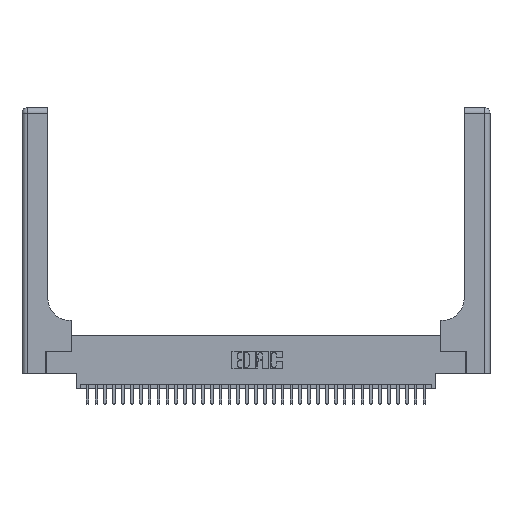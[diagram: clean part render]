
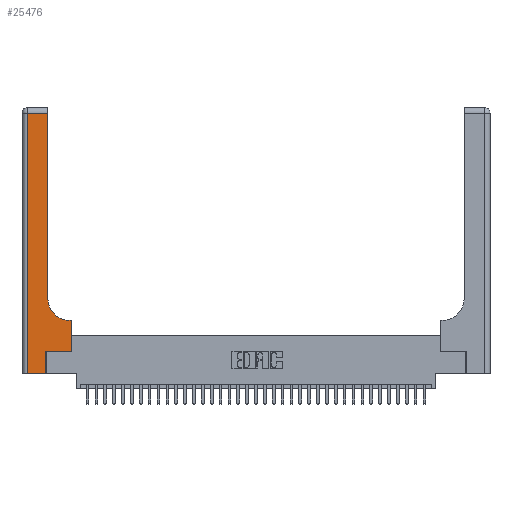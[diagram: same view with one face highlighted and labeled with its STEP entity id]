
A CAD part, top view. The second image highlights one B-rep face of the part: STEP entity #25476.
In plain terms, the highlighted planar face has unit normal (0, 0, 1).
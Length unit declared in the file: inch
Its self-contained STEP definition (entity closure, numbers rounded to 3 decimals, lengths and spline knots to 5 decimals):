
#682 = LINE ( 'NONE', #1012, #7306 ) ;
#921 = AXIS2_PLACEMENT_3D ( 'NONE', #27004, #12990, #32639 ) ;
#1012 = CARTESIAN_POINT ( 'NONE',  ( 0.2915, 3., 0.37 ) ) ;
#1309 = EDGE_CURVE ( 'NONE', #11380, #30281, #19876, .T. ) ;
#1618 = DIRECTION ( 'NONE',  ( 1., 0., 0. ) ) ;
#1779 = VECTOR ( 'NONE', #8010, 39.37008 ) ;
#2393 = CARTESIAN_POINT ( 'NONE',  ( 0.5585, 0.25, 0.37 ) ) ;
#2416 = DIRECTION ( 'NONE',  ( 0., -1., 0. ) ) ;
#2520 = ORIENTED_EDGE ( 'NONE', *, *, #9135, .T. ) ;
#3308 = DIRECTION ( 'NONE',  ( 0., 0., -1. ) ) ;
#3802 = CARTESIAN_POINT ( 'NONE',  ( 0.5585, 0.25, 0.37 ) ) ;
#3837 = ORIENTED_EDGE ( 'NONE', *, *, #32052, .T. ) ;
#4139 = DIRECTION ( 'NONE',  ( -1., 0., 0. ) ) ;
#5267 = CARTESIAN_POINT ( 'NONE',  ( 0.06, 3., 0.37 ) ) ;
#5445 = VECTOR ( 'NONE', #26536, 39.37008 ) ;
#5626 = ORIENTED_EDGE ( 'NONE', *, *, #15246, .T. ) ;
#5880 = CARTESIAN_POINT ( 'NONE',  ( 0.06, 2.94, 0.37 ) ) ;
#6284 = CARTESIAN_POINT ( 'NONE',  ( 0.2915, 0.6, 0.37 ) ) ;
#6336 = LINE ( 'NONE', #29250, #5445 ) ;
#6402 = VECTOR ( 'NONE', #23160, 39.37008 ) ;
#6829 = LINE ( 'NONE', #23845, #20947 ) ;
#7274 = LINE ( 'NONE', #6284, #6402 ) ;
#7306 = VECTOR ( 'NONE', #20758, 39.37008 ) ;
#7370 = ORIENTED_EDGE ( 'NONE', *, *, #23481, .T. ) ;
#7525 = CARTESIAN_POINT ( 'NONE',  ( 0.5585, 0.6, 0.37 ) ) ;
#8010 = DIRECTION ( 'NONE',  ( 0., 1., 0. ) ) ;
#8608 = LINE ( 'NONE', #5267, #14362 ) ;
#9135 = EDGE_CURVE ( 'NONE', #13445, #11380, #7274, .T. ) ;
#10134 = PLANE ( 'NONE',  #921 ) ;
#10916 = VECTOR ( 'NONE', #1618, 39.37008 ) ;
#11380 = VERTEX_POINT ( 'NONE', #29213 ) ;
#11761 = VERTEX_POINT ( 'NONE', #22426 ) ;
#11814 = ORIENTED_EDGE ( 'NONE', *, *, #1309, .T. ) ;
#12027 = VERTEX_POINT ( 'NONE', #3802 ) ;
#12164 = CARTESIAN_POINT ( 'NONE',  ( 0.06, 0., 0.37 ) ) ;
#12613 = CARTESIAN_POINT ( 'NONE',  ( 0.269, 0., 0.37 ) ) ;
#12990 = DIRECTION ( 'NONE',  ( 0., 0., -1. ) ) ;
#13445 = VERTEX_POINT ( 'NONE', #7525 ) ;
#13606 = LINE ( 'NONE', #2393, #19320 ) ;
#14362 = VECTOR ( 'NONE', #2416, 39.37008 ) ;
#15246 = EDGE_CURVE ( 'NONE', #32598, #11761, #23380, .T. ) ;
#16219 = ORIENTED_EDGE ( 'NONE', *, *, #24692, .T. ) ;
#16416 = CARTESIAN_POINT ( 'NONE',  ( 0.2915, 2.94, 0.37 ) ) ;
#16473 = DIRECTION ( 'NONE',  ( 0., 1., 0. ) ) ;
#16899 = EDGE_CURVE ( 'NONE', #30281, #21773, #682, .T. ) ;
#18358 = EDGE_CURVE ( 'NONE', #36426, #20912, #8608, .T. ) ;
#18532 = CARTESIAN_POINT ( 'NONE',  ( 0.269, 0.25, 0.37 ) ) ;
#19320 = VECTOR ( 'NONE', #16473, 39.37008 ) ;
#19876 = CIRCLE ( 'NONE', #35828, 0.25 ) ;
#20212 = CARTESIAN_POINT ( 'NONE',  ( 0.5415, 0.85, 0.37 ) ) ;
#20758 = DIRECTION ( 'NONE',  ( 0., 1., 0. ) ) ;
#20912 = VERTEX_POINT ( 'NONE', #12164 ) ;
#20947 = VECTOR ( 'NONE', #4139, 39.37008 ) ;
#21773 = VERTEX_POINT ( 'NONE', #16416 ) ;
#21905 = EDGE_LOOP ( 'NONE', ( #33339, #16219, #25431, #3837, #5626, #7370, #31620, #2520, #11814 ) ) ;
#22426 = CARTESIAN_POINT ( 'NONE',  ( 0.269, 0.25, 0.37 ) ) ;
#23040 = DIRECTION ( 'NONE',  ( 1., 0., 0. ) ) ;
#23160 = DIRECTION ( 'NONE',  ( -1., 0., 0. ) ) ;
#23380 = LINE ( 'NONE', #24863, #1779 ) ;
#23481 = EDGE_CURVE ( 'NONE', #11761, #12027, #24992, .T. ) ;
#23845 = CARTESIAN_POINT ( 'NONE',  ( 0., 2.94, 0.37 ) ) ;
#24408 = FACE_OUTER_BOUND ( 'NONE', #21905, .T. ) ;
#24692 = EDGE_CURVE ( 'NONE', #21773, #36426, #6829, .T. ) ;
#24863 = CARTESIAN_POINT ( 'NONE',  ( 0.269, 0., 0.37 ) ) ;
#24992 = LINE ( 'NONE', #18532, #10916 ) ;
#25431 = ORIENTED_EDGE ( 'NONE', *, *, #18358, .T. ) ;
#25476 = ADVANCED_FACE ( 'NONE', ( #24408 ), #10134, .F. ) ;
#26536 = DIRECTION ( 'NONE',  ( 1., 0., 0. ) ) ;
#27004 = CARTESIAN_POINT ( 'NONE',  ( 0., 3., 0.37 ) ) ;
#29213 = CARTESIAN_POINT ( 'NONE',  ( 0.5415, 0.6, 0.37 ) ) ;
#29250 = CARTESIAN_POINT ( 'NONE',  ( 0., 0., 0.37 ) ) ;
#29610 = EDGE_CURVE ( 'NONE', #12027, #13445, #13606, .T. ) ;
#30281 = VERTEX_POINT ( 'NONE', #30804 ) ;
#30804 = CARTESIAN_POINT ( 'NONE',  ( 0.2915, 0.85, 0.37 ) ) ;
#31620 = ORIENTED_EDGE ( 'NONE', *, *, #29610, .T. ) ;
#32052 = EDGE_CURVE ( 'NONE', #20912, #32598, #6336, .T. ) ;
#32598 = VERTEX_POINT ( 'NONE', #12613 ) ;
#32639 = DIRECTION ( 'NONE',  ( -1., 0., 0. ) ) ;
#33339 = ORIENTED_EDGE ( 'NONE', *, *, #16899, .T. ) ;
#35828 = AXIS2_PLACEMENT_3D ( 'NONE', #20212, #3308, #23040 ) ;
#36426 = VERTEX_POINT ( 'NONE', #5880 ) ;
